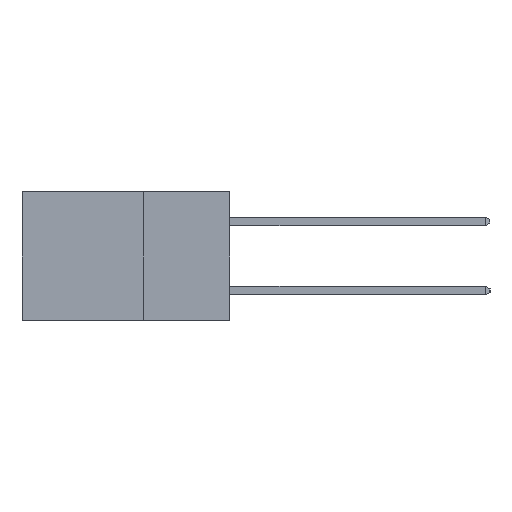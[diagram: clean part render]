
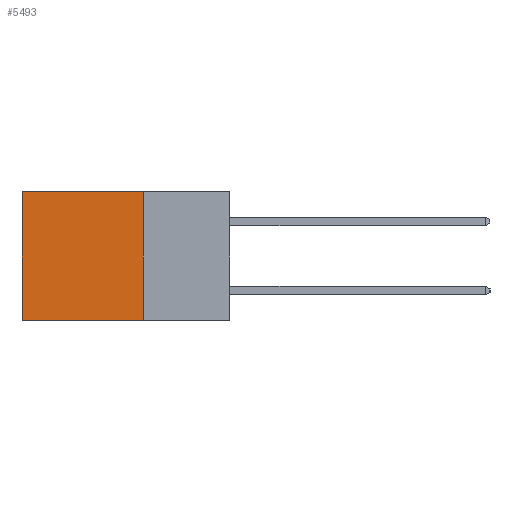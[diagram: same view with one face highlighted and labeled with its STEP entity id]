
A CAD part, left-side view. The second image highlights one B-rep face of the part: STEP entity #5493.
In plain terms, the highlighted planar face has unit normal (-1, 0, 0).
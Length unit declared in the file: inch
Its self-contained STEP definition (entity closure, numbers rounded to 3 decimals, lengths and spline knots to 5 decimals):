
#93 = VERTEX_POINT ( 'NONE', #2084 ) ;
#658 = CARTESIAN_POINT ( 'NONE',  ( 0.2615, 0.6, -0.37 ) ) ;
#1465 = VECTOR ( 'NONE', #15698, 39.37008 ) ;
#1507 = DIRECTION ( 'NONE',  ( 0., 1., 0. ) ) ;
#2084 = CARTESIAN_POINT ( 'NONE',  ( 0.2615, 0.6, 0. ) ) ;
#2129 = DIRECTION ( 'NONE',  ( 0., 0., -1. ) ) ;
#2387 = EDGE_CURVE ( 'NONE', #93, #2673, #16157, .T. ) ;
#2673 = VERTEX_POINT ( 'NONE', #19434 ) ;
#2917 = CARTESIAN_POINT ( 'NONE',  ( 0.2615, 0.25, -0.37 ) ) ;
#3277 = ORIENTED_EDGE ( 'NONE', *, *, #9046, .T. ) ;
#3582 = LINE ( 'NONE', #15969, #20971 ) ;
#5493 = ADVANCED_FACE ( 'NONE', ( #8776 ), #13031, .F. ) ;
#6327 = DIRECTION ( 'NONE',  ( 1., 0., 0. ) ) ;
#6666 = ORIENTED_EDGE ( 'NONE', *, *, #16853, .F. ) ;
#6795 = ORIENTED_EDGE ( 'NONE', *, *, #2387, .T. ) ;
#8776 = FACE_OUTER_BOUND ( 'NONE', #14926, .T. ) ;
#8898 = CARTESIAN_POINT ( 'NONE',  ( 0.2615, 0.25, 0. ) ) ;
#9046 = EDGE_CURVE ( 'NONE', #13752, #93, #10468, .T. ) ;
#9903 = EDGE_CURVE ( 'NONE', #13752, #17369, #3582, .T. ) ;
#10468 = LINE ( 'NONE', #8898, #1465 ) ;
#11398 = AXIS2_PLACEMENT_3D ( 'NONE', #2917, #6327, #18119 ) ;
#11604 = VECTOR ( 'NONE', #2129, 39.37008 ) ;
#13031 = PLANE ( 'NONE',  #11398 ) ;
#13120 = CARTESIAN_POINT ( 'NONE',  ( 0.2615, 0.25, 0. ) ) ;
#13549 = VECTOR ( 'NONE', #1507, 39.37008 ) ;
#13752 = VERTEX_POINT ( 'NONE', #13120 ) ;
#14926 = EDGE_LOOP ( 'NONE', ( #6795, #6666, #15967, #3277 ) ) ;
#15671 = CARTESIAN_POINT ( 'NONE',  ( 0.2615, 0.25, -0.37 ) ) ;
#15698 = DIRECTION ( 'NONE',  ( 0., 1., 0. ) ) ;
#15967 = ORIENTED_EDGE ( 'NONE', *, *, #9903, .F. ) ;
#15969 = CARTESIAN_POINT ( 'NONE',  ( 0.2615, 0.25, -0.37 ) ) ;
#16157 = LINE ( 'NONE', #658, #11604 ) ;
#16691 = CARTESIAN_POINT ( 'NONE',  ( 0.2615, 0.25, -0.37 ) ) ;
#16853 = EDGE_CURVE ( 'NONE', #17369, #2673, #18043, .T. ) ;
#17369 = VERTEX_POINT ( 'NONE', #15671 ) ;
#17631 = DIRECTION ( 'NONE',  ( 0., 0., -1. ) ) ;
#18043 = LINE ( 'NONE', #16691, #13549 ) ;
#18119 = DIRECTION ( 'NONE',  ( 0., 0., -1. ) ) ;
#19434 = CARTESIAN_POINT ( 'NONE',  ( 0.2615, 0.6, -0.37 ) ) ;
#20971 = VECTOR ( 'NONE', #17631, 39.37008 ) ;
